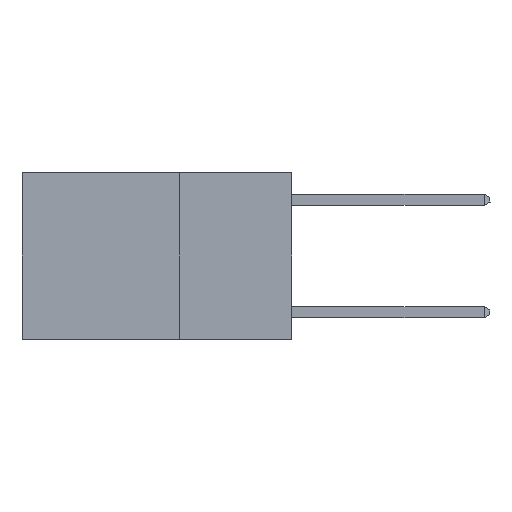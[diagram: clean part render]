
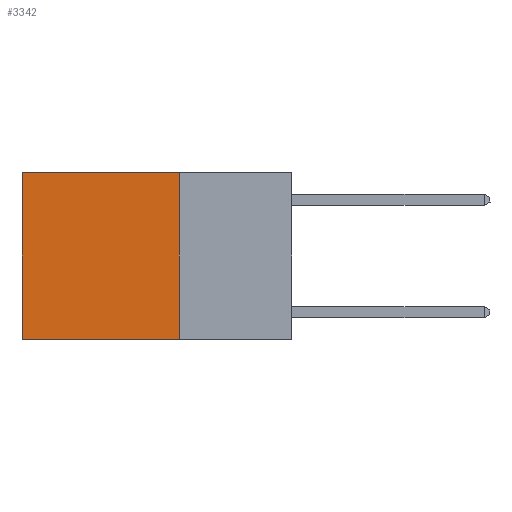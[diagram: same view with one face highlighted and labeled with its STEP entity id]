
A CAD part, left-side view. The second image highlights one B-rep face of the part: STEP entity #3342.
In plain terms, the highlighted planar face has unit normal (-1, 0, 0).
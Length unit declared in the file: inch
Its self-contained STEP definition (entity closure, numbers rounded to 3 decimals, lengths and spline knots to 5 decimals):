
#400 = PLANE ( 'NONE',  #9893 ) ;
#546 = VERTEX_POINT ( 'NONE', #15631 ) ;
#795 = VECTOR ( 'NONE', #8682, 39.37008 ) ;
#1187 = EDGE_CURVE ( 'NONE', #14100, #7289, #7119, .T. ) ;
#1381 = VECTOR ( 'NONE', #12022, 39.37008 ) ;
#1869 = ORIENTED_EDGE ( 'NONE', *, *, #1187, .F. ) ;
#2046 = EDGE_LOOP ( 'NONE', ( #10904, #14670, #1869, #6408 ) ) ;
#3104 = DIRECTION ( 'NONE',  ( 0., 0., -1. ) ) ;
#3342 = ADVANCED_FACE ( 'NONE', ( #7719 ), #400, .F. ) ;
#4621 = CARTESIAN_POINT ( 'NONE',  ( 0.2625, 0.25, -0.37 ) ) ;
#5133 = CARTESIAN_POINT ( 'NONE',  ( 0.2625, 0.25, 0. ) ) ;
#5229 = LINE ( 'NONE', #4621, #1381 ) ;
#6408 = ORIENTED_EDGE ( 'NONE', *, *, #15232, .T. ) ;
#6865 = EDGE_CURVE ( 'NONE', #7652, #546, #7639, .T. ) ;
#7119 = LINE ( 'NONE', #13733, #13257 ) ;
#7289 = VERTEX_POINT ( 'NONE', #15391 ) ;
#7436 = CARTESIAN_POINT ( 'NONE',  ( 0.2625, 0.6, 0. ) ) ;
#7639 = LINE ( 'NONE', #7436, #795 ) ;
#7652 = VERTEX_POINT ( 'NONE', #9219 ) ;
#7719 = FACE_OUTER_BOUND ( 'NONE', #2046, .T. ) ;
#7855 = EDGE_CURVE ( 'NONE', #7289, #546, #5229, .T. ) ;
#8657 = VECTOR ( 'NONE', #15284, 39.37008 ) ;
#8682 = DIRECTION ( 'NONE',  ( 0., 0., -1. ) ) ;
#9016 = LINE ( 'NONE', #9222, #8657 ) ;
#9219 = CARTESIAN_POINT ( 'NONE',  ( 0.2625, 0.6, 0. ) ) ;
#9222 = CARTESIAN_POINT ( 'NONE',  ( 0.2625, 0.25, 0. ) ) ;
#9329 = CARTESIAN_POINT ( 'NONE',  ( 0.2625, 0.25, 0. ) ) ;
#9893 = AXIS2_PLACEMENT_3D ( 'NONE', #9329, #10563, #3104 ) ;
#10563 = DIRECTION ( 'NONE',  ( 1., 0., 0. ) ) ;
#10904 = ORIENTED_EDGE ( 'NONE', *, *, #6865, .T. ) ;
#12022 = DIRECTION ( 'NONE',  ( 0., 1., 0. ) ) ;
#12516 = DIRECTION ( 'NONE',  ( 0., 0., -1. ) ) ;
#13257 = VECTOR ( 'NONE', #12516, 39.37008 ) ;
#13733 = CARTESIAN_POINT ( 'NONE',  ( 0.2625, 0.25, 0. ) ) ;
#14100 = VERTEX_POINT ( 'NONE', #5133 ) ;
#14670 = ORIENTED_EDGE ( 'NONE', *, *, #7855, .F. ) ;
#15232 = EDGE_CURVE ( 'NONE', #14100, #7652, #9016, .T. ) ;
#15284 = DIRECTION ( 'NONE',  ( 0., 1., 0. ) ) ;
#15391 = CARTESIAN_POINT ( 'NONE',  ( 0.2625, 0.25, -0.37 ) ) ;
#15631 = CARTESIAN_POINT ( 'NONE',  ( 0.2625, 0.6, -0.37 ) ) ;
